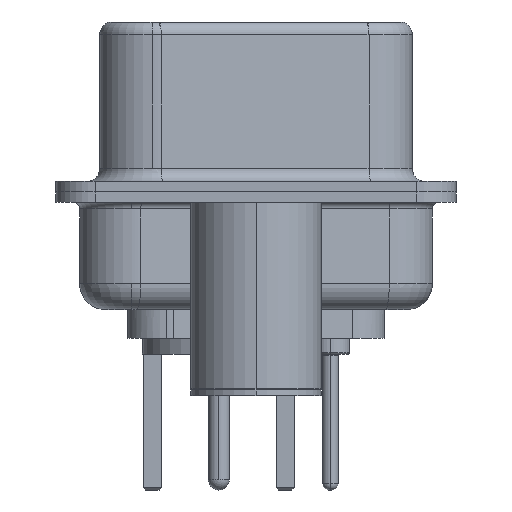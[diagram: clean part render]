
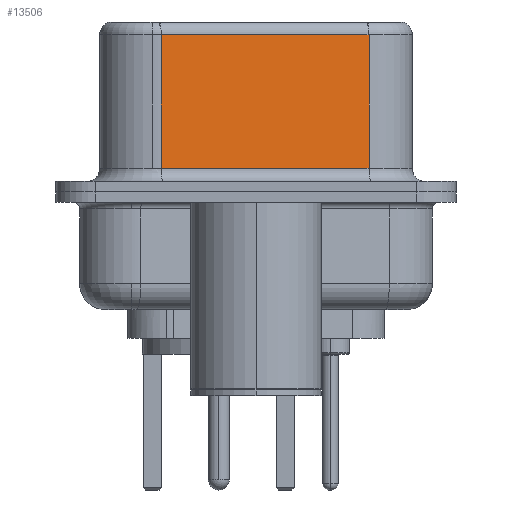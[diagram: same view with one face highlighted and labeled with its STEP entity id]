
A CAD part, left-side view. The second image highlights one B-rep face of the part: STEP entity #13506.
In plain terms, the highlighted planar face has unit normal (-0.985, -0.174, 0).
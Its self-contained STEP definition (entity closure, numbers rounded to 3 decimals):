
#265 = EDGE_CURVE ( 'NONE', #20957, #2646, #542, .T. ) ;
#400 = CARTESIAN_POINT ( 'NONE',  ( 5.132, -4.322, 6.52 ) ) ;
#542 = LINE ( 'NONE', #18727, #9997 ) ;
#1078 = DIRECTION ( 'NONE',  ( 0.174, -0.985, 0. ) ) ;
#2646 = VERTEX_POINT ( 'NONE', #22428 ) ;
#3281 = VERTEX_POINT ( 'NONE', #20800 ) ;
#4582 = PLANE ( 'NONE',  #7418 ) ;
#4823 = CARTESIAN_POINT ( 'NONE',  ( 3.73, 3.628, 6.52 ) ) ;
#7254 = DIRECTION ( 'NONE',  ( -0.174, 0.985, 0. ) ) ;
#7418 = AXIS2_PLACEMENT_3D ( 'NONE', #8361, #21491, #10238 ) ;
#8361 = CARTESIAN_POINT ( 'NONE',  ( 5.132, -4.322, 6.52 ) ) ;
#8703 = ORIENTED_EDGE ( 'NONE', *, *, #13409, .F. ) ;
#9983 = EDGE_LOOP ( 'NONE', ( #8703, #18122, #14898, #19366 ) ) ;
#9997 = VECTOR ( 'NONE', #1078, 1000. ) ;
#10238 = DIRECTION ( 'NONE',  ( -0.174, 0.985, 0. ) ) ;
#11613 = VECTOR ( 'NONE', #23558, 1000. ) ;
#11718 = DIRECTION ( 'NONE',  ( 0., 0., -1. ) ) ;
#12560 = FACE_OUTER_BOUND ( 'NONE', #9983, .T. ) ;
#13409 = EDGE_CURVE ( 'NONE', #3281, #2646, #21110, .T. ) ;
#13497 = VERTEX_POINT ( 'NONE', #15791 ) ;
#13506 = ADVANCED_FACE ( 'NONE', ( #12560 ), #4582, .F. ) ;
#13931 = VECTOR ( 'NONE', #7254, 1000. ) ;
#14898 = ORIENTED_EDGE ( 'NONE', *, *, #15552, .T. ) ;
#15552 = EDGE_CURVE ( 'NONE', #13497, #20957, #22196, .T. ) ;
#15791 = CARTESIAN_POINT ( 'NONE',  ( 3.73, 3.628, 6.02 ) ) ;
#16576 = EDGE_CURVE ( 'NONE', #3281, #13497, #18919, .T. ) ;
#16647 = CARTESIAN_POINT ( 'NONE',  ( 5.132, -4.322, 6.02 ) ) ;
#18122 = ORIENTED_EDGE ( 'NONE', *, *, #16576, .T. ) ;
#18727 = CARTESIAN_POINT ( 'NONE',  ( 5.132, -4.322, 0.9 ) ) ;
#18919 = LINE ( 'NONE', #16647, #13931 ) ;
#19366 = ORIENTED_EDGE ( 'NONE', *, *, #265, .T. ) ;
#20736 = CARTESIAN_POINT ( 'NONE',  ( 3.73, 3.628, 0.9 ) ) ;
#20800 = CARTESIAN_POINT ( 'NONE',  ( 5.132, -4.322, 6.02 ) ) ;
#20957 = VERTEX_POINT ( 'NONE', #20736 ) ;
#21110 = LINE ( 'NONE', #400, #24361 ) ;
#21491 = DIRECTION ( 'NONE',  ( 0.985, 0.174, 0. ) ) ;
#22196 = LINE ( 'NONE', #4823, #11613 ) ;
#22428 = CARTESIAN_POINT ( 'NONE',  ( 5.132, -4.322, 0.9 ) ) ;
#23558 = DIRECTION ( 'NONE',  ( 0., 0., -1. ) ) ;
#24361 = VECTOR ( 'NONE', #11718, 1000. ) ;
